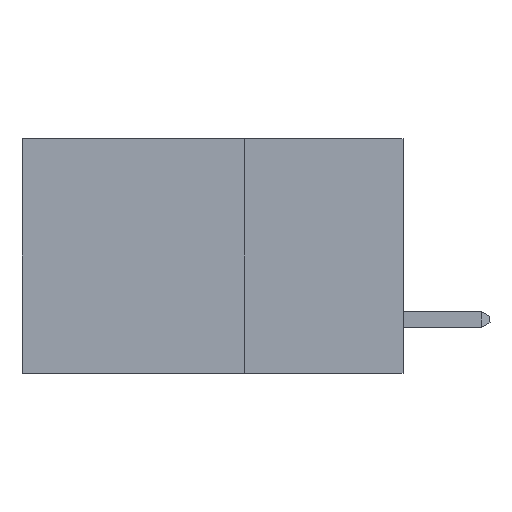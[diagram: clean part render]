
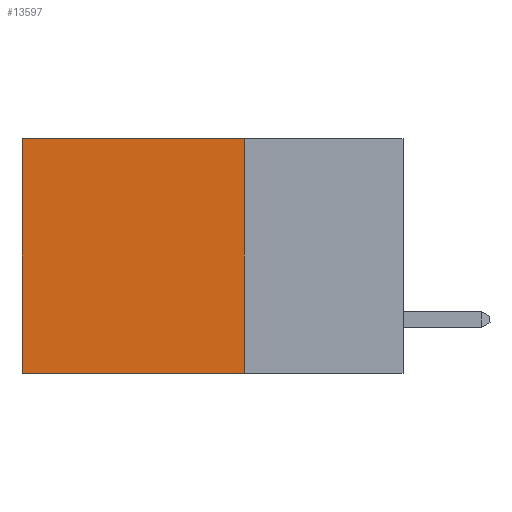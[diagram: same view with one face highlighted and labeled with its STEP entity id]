
A CAD part, left-side view. The second image highlights one B-rep face of the part: STEP entity #13597.
In plain terms, the highlighted planar face has unit normal (-1, 0, 0).
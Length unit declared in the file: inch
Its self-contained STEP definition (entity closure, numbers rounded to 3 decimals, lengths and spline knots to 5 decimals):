
#2487 = CARTESIAN_POINT ( 'NONE',  ( 0.2875, 0.25, 0. ) ) ;
#2622 = EDGE_CURVE ( 'NONE', #13790, #14483, #10254, .T. ) ;
#3035 = CARTESIAN_POINT ( 'NONE',  ( 0.2875, 0.25, -0.37 ) ) ;
#3337 = CARTESIAN_POINT ( 'NONE',  ( 0.2875, 0.25, 0. ) ) ;
#3530 = CARTESIAN_POINT ( 'NONE',  ( 0.2875, 0.25, 0. ) ) ;
#3591 = PLANE ( 'NONE',  #16066 ) ;
#3708 = CARTESIAN_POINT ( 'NONE',  ( 0.2875, 0.6, 0. ) ) ;
#4508 = ORIENTED_EDGE ( 'NONE', *, *, #10233, .F. ) ;
#4598 = VERTEX_POINT ( 'NONE', #5497 ) ;
#4921 = DIRECTION ( 'NONE',  ( 1., 0., 0. ) ) ;
#5497 = CARTESIAN_POINT ( 'NONE',  ( 0.2875, 0.25, -0.37 ) ) ;
#5619 = VECTOR ( 'NONE', #11188, 39.37008 ) ;
#5762 = ORIENTED_EDGE ( 'NONE', *, *, #14201, .F. ) ;
#6109 = LINE ( 'NONE', #3035, #11781 ) ;
#7034 = VECTOR ( 'NONE', #8545, 39.37008 ) ;
#8360 = CARTESIAN_POINT ( 'NONE',  ( 0.2875, 0.6, -0.37 ) ) ;
#8545 = DIRECTION ( 'NONE',  ( 0., 1., 0. ) ) ;
#8599 = EDGE_LOOP ( 'NONE', ( #12881, #5762, #4508, #15737 ) ) ;
#8846 = CARTESIAN_POINT ( 'NONE',  ( 0.2875, 0.25, 0. ) ) ;
#9016 = LINE ( 'NONE', #3708, #5619 ) ;
#9498 = DIRECTION ( 'NONE',  ( 0., 1., 0. ) ) ;
#9847 = LINE ( 'NONE', #3337, #15626 ) ;
#10233 = EDGE_CURVE ( 'NONE', #13790, #4598, #9847, .T. ) ;
#10254 = LINE ( 'NONE', #8846, #7034 ) ;
#11188 = DIRECTION ( 'NONE',  ( 0., 0., -1. ) ) ;
#11781 = VECTOR ( 'NONE', #9498, 39.37008 ) ;
#12881 = ORIENTED_EDGE ( 'NONE', *, *, #16188, .T. ) ;
#13205 = DIRECTION ( 'NONE',  ( 0., 0., -1. ) ) ;
#13259 = VERTEX_POINT ( 'NONE', #8360 ) ;
#13431 = DIRECTION ( 'NONE',  ( 0., 0., -1. ) ) ;
#13597 = ADVANCED_FACE ( 'NONE', ( #13601 ), #3591, .F. ) ;
#13601 = FACE_OUTER_BOUND ( 'NONE', #8599, .T. ) ;
#13790 = VERTEX_POINT ( 'NONE', #2487 ) ;
#14201 = EDGE_CURVE ( 'NONE', #4598, #13259, #6109, .T. ) ;
#14483 = VERTEX_POINT ( 'NONE', #15619 ) ;
#15619 = CARTESIAN_POINT ( 'NONE',  ( 0.2875, 0.6, 0. ) ) ;
#15626 = VECTOR ( 'NONE', #13205, 39.37008 ) ;
#15737 = ORIENTED_EDGE ( 'NONE', *, *, #2622, .T. ) ;
#16066 = AXIS2_PLACEMENT_3D ( 'NONE', #3530, #4921, #13431 ) ;
#16188 = EDGE_CURVE ( 'NONE', #14483, #13259, #9016, .T. ) ;
